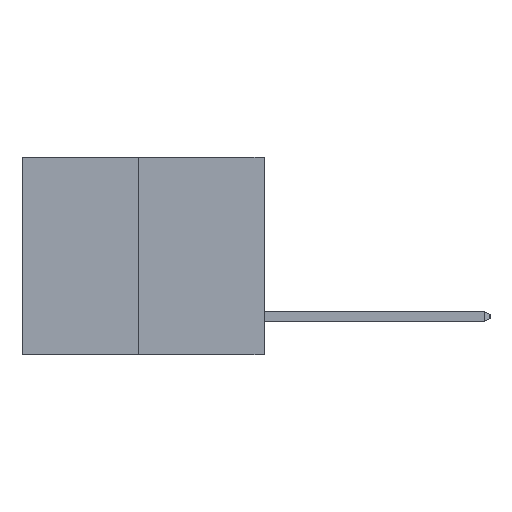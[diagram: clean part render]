
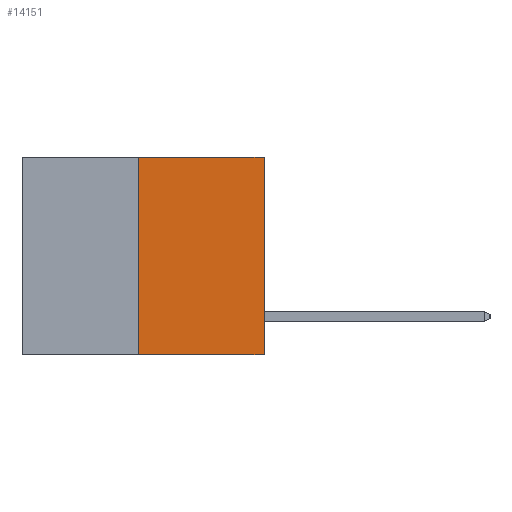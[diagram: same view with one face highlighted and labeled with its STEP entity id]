
A CAD part, left-side view. The second image highlights one B-rep face of the part: STEP entity #14151.
In plain terms, the highlighted planar face has unit normal (-1, 0, 0).
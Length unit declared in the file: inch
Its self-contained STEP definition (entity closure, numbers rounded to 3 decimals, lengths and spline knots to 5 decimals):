
#3169 = EDGE_CURVE ( 'NONE', #5485, #6362, #16724, .T. ) ;
#3689 = EDGE_CURVE ( 'NONE', #8883, #5485, #13285, .T. ) ;
#3913 = ORIENTED_EDGE ( 'NONE', *, *, #5781, .F. ) ;
#4043 = CARTESIAN_POINT ( 'NONE',  ( 0., 0.6, -0.49 ) ) ;
#4876 = PLANE ( 'NONE',  #9500 ) ;
#5126 = DIRECTION ( 'NONE',  ( 0., 0., 1. ) ) ;
#5485 = VERTEX_POINT ( 'NONE', #15354 ) ;
#5781 = EDGE_CURVE ( 'NONE', #8883, #11629, #8622, .T. ) ;
#6314 = DIRECTION ( 'NONE',  ( 1., 0., 0. ) ) ;
#6362 = VERTEX_POINT ( 'NONE', #8548 ) ;
#6889 = VECTOR ( 'NONE', #5126, 39.37008 ) ;
#6991 = EDGE_LOOP ( 'NONE', ( #3913, #7815, #16515, #15332 ) ) ;
#7348 = VECTOR ( 'NONE', #14816, 39.37008 ) ;
#7744 = LINE ( 'NONE', #10445, #7348 ) ;
#7815 = ORIENTED_EDGE ( 'NONE', *, *, #3689, .T. ) ;
#7940 = CARTESIAN_POINT ( 'NONE',  ( 0., 0.312, -0.49 ) ) ;
#8548 = CARTESIAN_POINT ( 'NONE',  ( 0., 0., 0. ) ) ;
#8622 = LINE ( 'NONE', #7940, #6889 ) ;
#8883 = VERTEX_POINT ( 'NONE', #12836 ) ;
#9344 = DIRECTION ( 'NONE',  ( 0., -1., 0. ) ) ;
#9383 = CARTESIAN_POINT ( 'NONE',  ( 0., 0.312, 0. ) ) ;
#9500 = AXIS2_PLACEMENT_3D ( 'NONE', #14633, #6314, #17552 ) ;
#9969 = CARTESIAN_POINT ( 'NONE',  ( 0., 0., 0. ) ) ;
#10099 = VECTOR ( 'NONE', #14044, 39.37008 ) ;
#10445 = CARTESIAN_POINT ( 'NONE',  ( 0., 0.6, 0. ) ) ;
#11629 = VERTEX_POINT ( 'NONE', #9383 ) ;
#12836 = CARTESIAN_POINT ( 'NONE',  ( 0., 0.312, -0.49 ) ) ;
#13014 = FACE_OUTER_BOUND ( 'NONE', #6991, .T. ) ;
#13285 = LINE ( 'NONE', #4043, #17074 ) ;
#14044 = DIRECTION ( 'NONE',  ( 0., 0., 1. ) ) ;
#14151 = ADVANCED_FACE ( 'NONE', ( #13014 ), #4876, .F. ) ;
#14633 = CARTESIAN_POINT ( 'NONE',  ( 0., 0.6, 0. ) ) ;
#14816 = DIRECTION ( 'NONE',  ( 0., -1., 0. ) ) ;
#15332 = ORIENTED_EDGE ( 'NONE', *, *, #17825, .F. ) ;
#15354 = CARTESIAN_POINT ( 'NONE',  ( 0., 0., -0.49 ) ) ;
#16515 = ORIENTED_EDGE ( 'NONE', *, *, #3169, .T. ) ;
#16724 = LINE ( 'NONE', #9969, #10099 ) ;
#17074 = VECTOR ( 'NONE', #9344, 39.37008 ) ;
#17552 = DIRECTION ( 'NONE',  ( 0., 0., -1. ) ) ;
#17825 = EDGE_CURVE ( 'NONE', #11629, #6362, #7744, .T. ) ;
